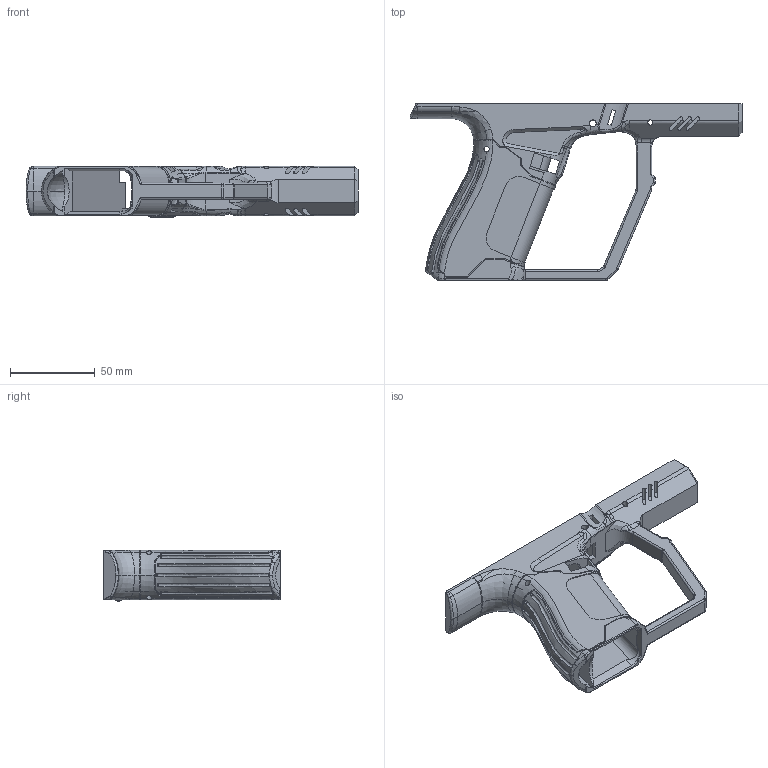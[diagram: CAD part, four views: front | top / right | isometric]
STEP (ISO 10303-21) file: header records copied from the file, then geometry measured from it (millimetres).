
FILE_DESCRIPTION(/* description */ (''),/* implementation_level */ '2;1');
FILE_NAME(/* name */ 'Halo Magnum Frame.step',/* time_stamp */ '2022-03-30T10:08:51-06:00',/* author */ (''),/* organization */ (''),/* preprocessor_version */ 'ST-DEVELOPER v18.1',/* originating_system */ 'Autodesk Translation Framework v10.14.0.1471',/* authorisation */ '');
FILE_SCHEMA (('AUTOMOTIVE_DESIGN { 1 0 10303 214 3 1 1 }'));
Products named in the file (1): Halo Magnum Beta
Bounding box: 196.02 x 104.35 x 30.3 mm (x, y, z)
Volume: 96374.1 mm3; surface area: 56362.8 mm2
Topology: 1 solids, 2 shells, 649 faces, 1887 edges, 1210 vertices
Faces by surface type: bspline 262, plane 237, cylinder 140, torus 10
Full cylindrical faces by diameter (mm): 1.522 x1, 1.904 x1, 3.13 x2, 3.147 x2, 4.11 x2
Entity records: 53179 total; most frequent: CARTESIAN_POINT 37756, ORIENTED_EDGE 3744, DIRECTION 2494, EDGE_CURVE 1872, VERTEX_POINT 1210, AXIS2_PLACEMENT_3D 845, LINE 804, VECTOR 804
